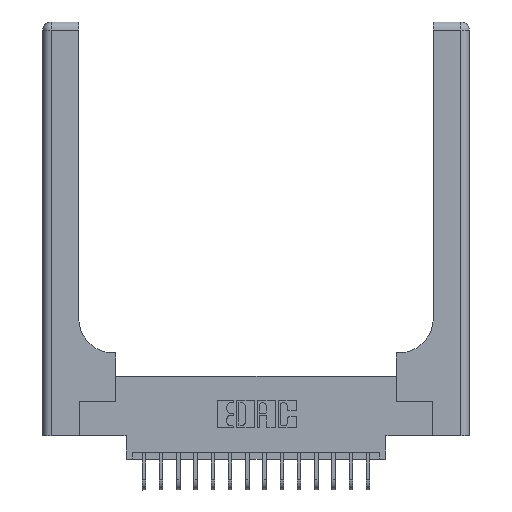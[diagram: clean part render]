
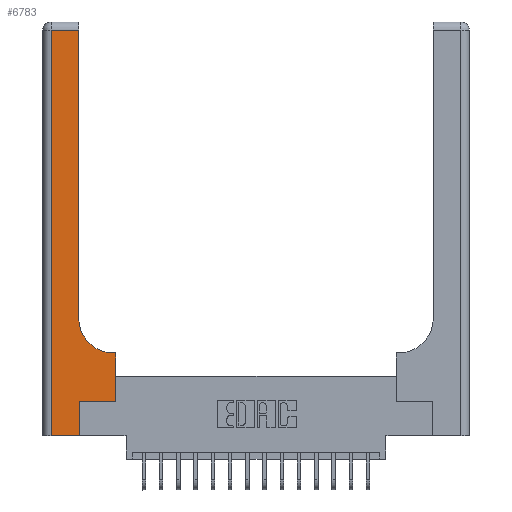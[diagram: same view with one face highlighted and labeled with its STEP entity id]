
A CAD part, top view. The second image highlights one B-rep face of the part: STEP entity #6783.
In plain terms, the highlighted planar face has unit normal (0, 0, 1).
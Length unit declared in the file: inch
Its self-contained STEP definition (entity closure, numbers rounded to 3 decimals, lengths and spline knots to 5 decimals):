
#785 = EDGE_CURVE ( 'NONE', #8450, #9286, #14212, .T. ) ;
#968 = CARTESIAN_POINT ( 'NONE',  ( 0.06, 2.94, 0.37 ) ) ;
#1025 = CARTESIAN_POINT ( 'NONE',  ( 0.06, 0., 0.37 ) ) ;
#1321 = VECTOR ( 'NONE', #17239, 39.37008 ) ;
#1573 = CARTESIAN_POINT ( 'NONE',  ( 0.265, 0., 0.37 ) ) ;
#2057 = ORIENTED_EDGE ( 'NONE', *, *, #785, .T. ) ;
#2346 = EDGE_CURVE ( 'NONE', #16603, #2827, #3004, .T. ) ;
#2644 = EDGE_LOOP ( 'NONE', ( #10297, #6249, #2057, #13061, #3630, #14082, #18960, #13289, #11031 ) ) ;
#2827 = VERTEX_POINT ( 'NONE', #17060 ) ;
#3004 = LINE ( 'NONE', #6216, #17692 ) ;
#3101 = EDGE_CURVE ( 'NONE', #14278, #16603, #13938, .T. ) ;
#3265 = VERTEX_POINT ( 'NONE', #7933 ) ;
#3630 = ORIENTED_EDGE ( 'NONE', *, *, #3101, .T. ) ;
#3988 = CARTESIAN_POINT ( 'NONE',  ( 0.528, 0.6, 0.37 ) ) ;
#4278 = EDGE_CURVE ( 'NONE', #2827, #17032, #10956, .T. ) ;
#4970 = DIRECTION ( 'NONE',  ( -1., 0., 0. ) ) ;
#5111 = VERTEX_POINT ( 'NONE', #17421 ) ;
#5273 = LINE ( 'NONE', #19063, #13941 ) ;
#6049 = CARTESIAN_POINT ( 'NONE',  ( 0.51, 0.85, 0.37 ) ) ;
#6216 = CARTESIAN_POINT ( 'NONE',  ( 0.265, 0.25, 0.37 ) ) ;
#6249 = ORIENTED_EDGE ( 'NONE', *, *, #12667, .T. ) ;
#6783 = ADVANCED_FACE ( 'NONE', ( #19700 ), #16591, .F. ) ;
#6992 = CARTESIAN_POINT ( 'NONE',  ( 0.26, 2.94, 0.37 ) ) ;
#7903 = CARTESIAN_POINT ( 'NONE',  ( 0.06, 3., 0.37 ) ) ;
#7933 = CARTESIAN_POINT ( 'NONE',  ( 0.26, 0.85, 0.37 ) ) ;
#8450 = VERTEX_POINT ( 'NONE', #968 ) ;
#8803 = VECTOR ( 'NONE', #10260, 39.37008 ) ;
#8958 = DIRECTION ( 'NONE',  ( 0., 1., 0. ) ) ;
#9286 = VERTEX_POINT ( 'NONE', #1025 ) ;
#9818 = EDGE_CURVE ( 'NONE', #5111, #3265, #9959, .T. ) ;
#9959 = CIRCLE ( 'NONE', #15590, 0.25 ) ;
#10260 = DIRECTION ( 'NONE',  ( 1., 0., 0. ) ) ;
#10297 = ORIENTED_EDGE ( 'NONE', *, *, #14944, .T. ) ;
#10708 = LINE ( 'NONE', #15376, #19957 ) ;
#10956 = LINE ( 'NONE', #15827, #19402 ) ;
#11031 = ORIENTED_EDGE ( 'NONE', *, *, #9818, .T. ) ;
#11191 = AXIS2_PLACEMENT_3D ( 'NONE', #15137, #13580, #16794 ) ;
#11796 = CARTESIAN_POINT ( 'NONE',  ( 0.26, 0.6, 0.37 ) ) ;
#12090 = CARTESIAN_POINT ( 'NONE',  ( 0.265, 0.25, 0.37 ) ) ;
#12667 = EDGE_CURVE ( 'NONE', #13530, #8450, #5273, .T. ) ;
#12853 = DIRECTION ( 'NONE',  ( 0., -1., 0. ) ) ;
#13061 = ORIENTED_EDGE ( 'NONE', *, *, #19952, .T. ) ;
#13289 = ORIENTED_EDGE ( 'NONE', *, *, #15657, .T. ) ;
#13530 = VERTEX_POINT ( 'NONE', #6992 ) ;
#13580 = DIRECTION ( 'NONE',  ( 0., 0., -1. ) ) ;
#13767 = VECTOR ( 'NONE', #12853, 39.37008 ) ;
#13938 = LINE ( 'NONE', #14139, #1321 ) ;
#13941 = VECTOR ( 'NONE', #4970, 39.37008 ) ;
#14082 = ORIENTED_EDGE ( 'NONE', *, *, #2346, .T. ) ;
#14139 = CARTESIAN_POINT ( 'NONE',  ( 0.265, 0., 0.37 ) ) ;
#14212 = LINE ( 'NONE', #7903, #13767 ) ;
#14270 = DIRECTION ( 'NONE',  ( 0., 1., 0. ) ) ;
#14278 = VERTEX_POINT ( 'NONE', #1573 ) ;
#14944 = EDGE_CURVE ( 'NONE', #3265, #13530, #10708, .T. ) ;
#15024 = VECTOR ( 'NONE', #16360, 39.37008 ) ;
#15137 = CARTESIAN_POINT ( 'NONE',  ( 0., 3., 0.37 ) ) ;
#15376 = CARTESIAN_POINT ( 'NONE',  ( 0.26, 3., 0.37 ) ) ;
#15590 = AXIS2_PLACEMENT_3D ( 'NONE', #6049, #17019, #18891 ) ;
#15657 = EDGE_CURVE ( 'NONE', #17032, #5111, #19780, .T. ) ;
#15827 = CARTESIAN_POINT ( 'NONE',  ( 0.528, 0.25, 0.37 ) ) ;
#15849 = DIRECTION ( 'NONE',  ( 1., 0., 0. ) ) ;
#16360 = DIRECTION ( 'NONE',  ( -1., 0., 0. ) ) ;
#16591 = PLANE ( 'NONE',  #11191 ) ;
#16603 = VERTEX_POINT ( 'NONE', #12090 ) ;
#16794 = DIRECTION ( 'NONE',  ( -1., 0., 0. ) ) ;
#17019 = DIRECTION ( 'NONE',  ( 0., 0., -1. ) ) ;
#17032 = VERTEX_POINT ( 'NONE', #3988 ) ;
#17060 = CARTESIAN_POINT ( 'NONE',  ( 0.528, 0.25, 0.37 ) ) ;
#17239 = DIRECTION ( 'NONE',  ( 0., 1., 0. ) ) ;
#17421 = CARTESIAN_POINT ( 'NONE',  ( 0.51, 0.6, 0.37 ) ) ;
#17692 = VECTOR ( 'NONE', #15849, 39.37008 ) ;
#18131 = LINE ( 'NONE', #18447, #8803 ) ;
#18447 = CARTESIAN_POINT ( 'NONE',  ( 0., 0., 0.37 ) ) ;
#18891 = DIRECTION ( 'NONE',  ( 1., 0., 0. ) ) ;
#18960 = ORIENTED_EDGE ( 'NONE', *, *, #4278, .T. ) ;
#19063 = CARTESIAN_POINT ( 'NONE',  ( 0., 2.94, 0.37 ) ) ;
#19402 = VECTOR ( 'NONE', #14270, 39.37008 ) ;
#19700 = FACE_OUTER_BOUND ( 'NONE', #2644, .T. ) ;
#19780 = LINE ( 'NONE', #11796, #15024 ) ;
#19952 = EDGE_CURVE ( 'NONE', #9286, #14278, #18131, .T. ) ;
#19957 = VECTOR ( 'NONE', #8958, 39.37008 ) ;
